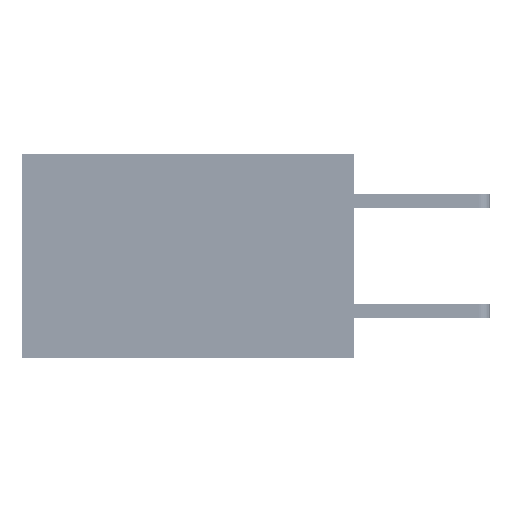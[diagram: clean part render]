
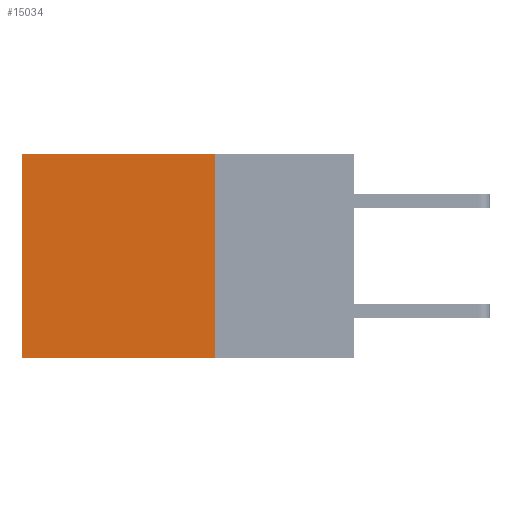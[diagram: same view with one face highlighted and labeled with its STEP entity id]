
A CAD part, left-side view. The second image highlights one B-rep face of the part: STEP entity #15034.
In plain terms, the highlighted planar face has unit normal (-1, 0, 0).
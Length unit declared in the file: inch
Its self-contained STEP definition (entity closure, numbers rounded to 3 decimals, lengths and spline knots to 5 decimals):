
#3898 = CARTESIAN_POINT ( 'NONE',  ( 0.2875, 0.25, 0. ) ) ;
#4707 = VERTEX_POINT ( 'NONE', #11844 ) ;
#5775 = VERTEX_POINT ( 'NONE', #17953 ) ;
#8870 = VERTEX_POINT ( 'NONE', #46667 ) ;
#11338 = LINE ( 'NONE', #14797, #26857 ) ;
#11545 = EDGE_CURVE ( 'NONE', #4707, #8870, #29753, .T. ) ;
#11844 = CARTESIAN_POINT ( 'NONE',  ( 0.2875, 0.25, 0. ) ) ;
#14162 = ORIENTED_EDGE ( 'NONE', *, *, #25784, .F. ) ;
#14359 = CARTESIAN_POINT ( 'NONE',  ( 0.2875, 0.25, 0. ) ) ;
#14797 = CARTESIAN_POINT ( 'NONE',  ( 0.2875, 0.25, -0.37 ) ) ;
#15034 = ADVANCED_FACE ( 'NONE', ( #28307 ), #41925, .F. ) ;
#15873 = VECTOR ( 'NONE', #29502, 39.37008 ) ;
#17165 = EDGE_CURVE ( 'NONE', #8870, #32987, #28679, .T. ) ;
#17953 = CARTESIAN_POINT ( 'NONE',  ( 0.2875, 0.25, -0.37 ) ) ;
#18034 = ORIENTED_EDGE ( 'NONE', *, *, #36654, .F. ) ;
#18272 = DIRECTION ( 'NONE',  ( 0., 0., -1. ) ) ;
#18865 = VECTOR ( 'NONE', #18272, 39.37008 ) ;
#19633 = VECTOR ( 'NONE', #26428, 39.37008 ) ;
#22461 = CARTESIAN_POINT ( 'NONE',  ( 0.2875, 0.6, 0. ) ) ;
#24322 = EDGE_LOOP ( 'NONE', ( #39657, #14162, #18034, #36313 ) ) ;
#25784 = EDGE_CURVE ( 'NONE', #5775, #32987, #11338, .T. ) ;
#26428 = DIRECTION ( 'NONE',  ( 0., 0., -1. ) ) ;
#26857 = VECTOR ( 'NONE', #40431, 39.37008 ) ;
#28307 = FACE_OUTER_BOUND ( 'NONE', #24322, .T. ) ;
#28535 = AXIS2_PLACEMENT_3D ( 'NONE', #38519, #34851, #30650 ) ;
#28679 = LINE ( 'NONE', #22461, #18865 ) ;
#29502 = DIRECTION ( 'NONE',  ( 0., 1., 0. ) ) ;
#29753 = LINE ( 'NONE', #14359, #15873 ) ;
#30650 = DIRECTION ( 'NONE',  ( 0., 0., -1. ) ) ;
#32987 = VERTEX_POINT ( 'NONE', #43071 ) ;
#34851 = DIRECTION ( 'NONE',  ( 1., 0., 0. ) ) ;
#36313 = ORIENTED_EDGE ( 'NONE', *, *, #11545, .T. ) ;
#36654 = EDGE_CURVE ( 'NONE', #4707, #5775, #45291, .T. ) ;
#38519 = CARTESIAN_POINT ( 'NONE',  ( 0.2875, 0.25, 0. ) ) ;
#39657 = ORIENTED_EDGE ( 'NONE', *, *, #17165, .T. ) ;
#40431 = DIRECTION ( 'NONE',  ( 0., 1., 0. ) ) ;
#41925 = PLANE ( 'NONE',  #28535 ) ;
#43071 = CARTESIAN_POINT ( 'NONE',  ( 0.2875, 0.6, -0.37 ) ) ;
#45291 = LINE ( 'NONE', #3898, #19633 ) ;
#46667 = CARTESIAN_POINT ( 'NONE',  ( 0.2875, 0.6, 0. ) ) ;
